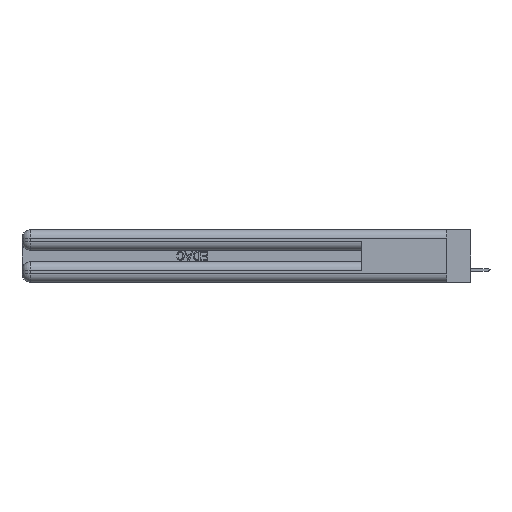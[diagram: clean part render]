
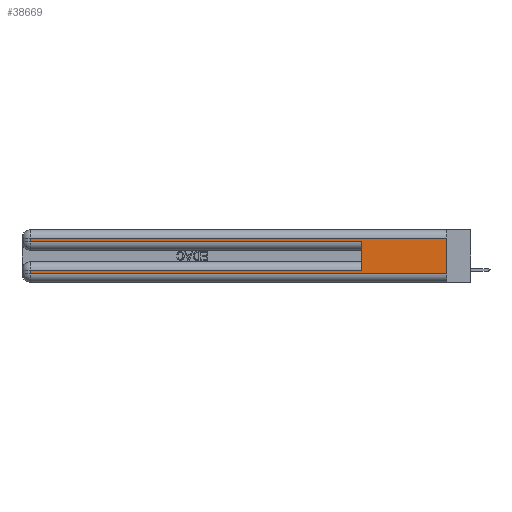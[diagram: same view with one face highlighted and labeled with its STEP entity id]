
A CAD part, left-side view. The second image highlights one B-rep face of the part: STEP entity #38669.
In plain terms, the highlighted planar face has unit normal (-1, 0, 0).
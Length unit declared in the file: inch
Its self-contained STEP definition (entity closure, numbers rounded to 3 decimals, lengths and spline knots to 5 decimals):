
#478 = PLANE ( 'NONE',  #35986 ) ;
#958 = EDGE_CURVE ( 'NONE', #31485, #15234, #15467, .T. ) ;
#1443 = CARTESIAN_POINT ( 'NONE',  ( 0., 2.94, 0.085 ) ) ;
#1618 = LINE ( 'NONE', #17210, #6663 ) ;
#1695 = LINE ( 'NONE', #35275, #35901 ) ;
#3246 = DIRECTION ( 'NONE',  ( 0., 1., 0. ) ) ;
#3931 = CARTESIAN_POINT ( 'NONE',  ( 0., 0., 0.31 ) ) ;
#4677 = VECTOR ( 'NONE', #21519, 39.37008 ) ;
#6005 = ORIENTED_EDGE ( 'NONE', *, *, #29518, .T. ) ;
#6479 = DIRECTION ( 'NONE',  ( 0., 0., -1. ) ) ;
#6547 = VECTOR ( 'NONE', #39443, 39.37008 ) ;
#6663 = VECTOR ( 'NONE', #35186, 39.37008 ) ;
#7136 = ORIENTED_EDGE ( 'NONE', *, *, #12100, .F. ) ;
#7823 = VECTOR ( 'NONE', #3246, 39.37008 ) ;
#8106 = VERTEX_POINT ( 'NONE', #39403 ) ;
#9955 = VECTOR ( 'NONE', #29639, 39.37008 ) ;
#11063 = VECTOR ( 'NONE', #6479, 39.37008 ) ;
#12100 = EDGE_CURVE ( 'NONE', #19032, #21364, #36264, .T. ) ;
#12858 = EDGE_CURVE ( 'NONE', #8106, #21018, #12865, .T. ) ;
#12862 = EDGE_CURVE ( 'NONE', #31485, #21018, #19082, .T. ) ;
#12865 = LINE ( 'NONE', #25098, #4677 ) ;
#13864 = CARTESIAN_POINT ( 'NONE',  ( 0., 0., 0.285 ) ) ;
#15087 = CARTESIAN_POINT ( 'NONE',  ( 0., 0.6, 0.145 ) ) ;
#15234 = VERTEX_POINT ( 'NONE', #22993 ) ;
#15467 = LINE ( 'NONE', #18274, #7823 ) ;
#17123 = VECTOR ( 'NONE', #33043, 39.37008 ) ;
#17210 = CARTESIAN_POINT ( 'NONE',  ( 0., 0., 0.085 ) ) ;
#17451 = EDGE_LOOP ( 'NONE', ( #38858, #24745, #30943, #19512, #7136, #6005, #29130, #25900 ) ) ;
#17454 = LINE ( 'NONE', #13864, #9955 ) ;
#18274 = CARTESIAN_POINT ( 'NONE',  ( 0., 0., 0.31 ) ) ;
#18462 = CARTESIAN_POINT ( 'NONE',  ( 0., 0., 0.37 ) ) ;
#19032 = VERTEX_POINT ( 'NONE', #30121 ) ;
#19082 = LINE ( 'NONE', #33865, #11063 ) ;
#19512 = ORIENTED_EDGE ( 'NONE', *, *, #33452, .T. ) ;
#19962 = EDGE_CURVE ( 'NONE', #37470, #8106, #39420, .T. ) ;
#21018 = VERTEX_POINT ( 'NONE', #31763 ) ;
#21364 = VERTEX_POINT ( 'NONE', #25528 ) ;
#21519 = DIRECTION ( 'NONE',  ( 0., -1., 0. ) ) ;
#21887 = DIRECTION ( 'NONE',  ( 0., 0., -1. ) ) ;
#22993 = CARTESIAN_POINT ( 'NONE',  ( 0., 2.94, 0.31 ) ) ;
#24745 = ORIENTED_EDGE ( 'NONE', *, *, #958, .T. ) ;
#25098 = CARTESIAN_POINT ( 'NONE',  ( 0., 0., 0.06 ) ) ;
#25528 = CARTESIAN_POINT ( 'NONE',  ( 0., 0.6, 0.285 ) ) ;
#25900 = ORIENTED_EDGE ( 'NONE', *, *, #12858, .T. ) ;
#26875 = CARTESIAN_POINT ( 'NONE',  ( 0., 2.94, 0.285 ) ) ;
#27858 = FACE_OUTER_BOUND ( 'NONE', #17451, .T. ) ;
#29130 = ORIENTED_EDGE ( 'NONE', *, *, #19962, .T. ) ;
#29518 = EDGE_CURVE ( 'NONE', #19032, #37470, #1618, .T. ) ;
#29639 = DIRECTION ( 'NONE',  ( 0., -1., 0. ) ) ;
#30121 = CARTESIAN_POINT ( 'NONE',  ( 0., 0.6, 0.085 ) ) ;
#30943 = ORIENTED_EDGE ( 'NONE', *, *, #37169, .T. ) ;
#31485 = VERTEX_POINT ( 'NONE', #3931 ) ;
#31763 = CARTESIAN_POINT ( 'NONE',  ( 0., 0., 0.06 ) ) ;
#33043 = DIRECTION ( 'NONE',  ( 0., 0., -1. ) ) ;
#33069 = VERTEX_POINT ( 'NONE', #26875 ) ;
#33257 = DIRECTION ( 'NONE',  ( 1., 0., 0. ) ) ;
#33452 = EDGE_CURVE ( 'NONE', #33069, #21364, #17454, .T. ) ;
#33865 = CARTESIAN_POINT ( 'NONE',  ( 0., 0., 0.37 ) ) ;
#35186 = DIRECTION ( 'NONE',  ( 0., 1., 0. ) ) ;
#35275 = CARTESIAN_POINT ( 'NONE',  ( 0., 2.94, 0.37 ) ) ;
#35901 = VECTOR ( 'NONE', #36073, 39.37008 ) ;
#35986 = AXIS2_PLACEMENT_3D ( 'NONE', #18462, #33257, #21887 ) ;
#36073 = DIRECTION ( 'NONE',  ( 0., 0., -1. ) ) ;
#36264 = LINE ( 'NONE', #15087, #6547 ) ;
#36643 = CARTESIAN_POINT ( 'NONE',  ( 0., 2.94, 0.37 ) ) ;
#37169 = EDGE_CURVE ( 'NONE', #15234, #33069, #1695, .T. ) ;
#37470 = VERTEX_POINT ( 'NONE', #1443 ) ;
#38669 = ADVANCED_FACE ( 'NONE', ( #27858 ), #478, .F. ) ;
#38858 = ORIENTED_EDGE ( 'NONE', *, *, #12862, .F. ) ;
#39403 = CARTESIAN_POINT ( 'NONE',  ( 0., 2.94, 0.06 ) ) ;
#39420 = LINE ( 'NONE', #36643, #17123 ) ;
#39443 = DIRECTION ( 'NONE',  ( 0., 0., 1. ) ) ;
